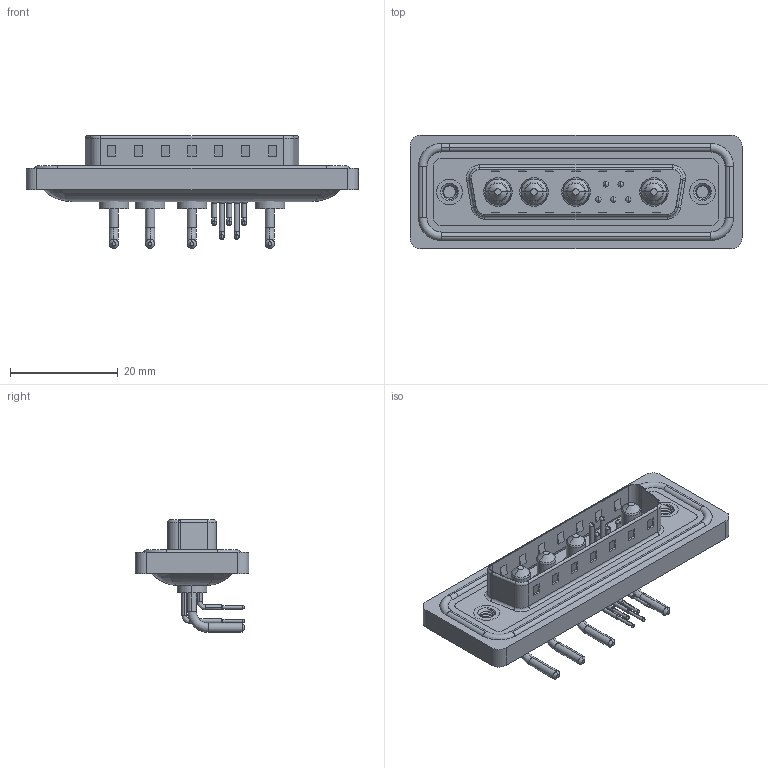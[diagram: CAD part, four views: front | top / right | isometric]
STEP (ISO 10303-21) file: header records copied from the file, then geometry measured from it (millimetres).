
FILE_DESCRIPTION (( 'STEP AP203' ), '1' );
FILE_NAME ('629W9W4-240-1N2.STEP', '2024-04-11T15:27:52', ( '' ), ( '' ), 'SwSTEP 2.0', 'SolidWorks 2023', '' );
FILE_SCHEMA (( 'CONFIG_CONTROL_DESIGN' ));
Length unit declared in the file: millimetre
Products named in the file (9): 629Combo Shell Front_25 Contacts; 629Combo Waterproof Housing_25 Contacts; 629Combo Threaded Rivet_2; 629Combo Shell Rear_25 Contacts; 629Combo Contact Row 1; 629Combo Housing_9W4; 629Combo Contact Row 2; Power Pin_10A RA; 629W9W4-240-1N2
Assembly tree (15 placements, depth 2):
  629W9W4-240-1N2
    629Combo Housing_9W4
    629Combo Shell Rear_25 Contacts
    629Combo Shell Front_25 Contacts
    629Combo Waterproof Housing_25 Contacts
    629Combo Threaded Rivet_2  x2
    Power Pin_10A RA  x4
    629Combo Contact Row 1  x2
    629Combo Contact Row 2  x3
Bounding box: 61.75 x 21.1 x 20.95 mm (x, y, z)
Volume: 7483.2 mm3; surface area: 12173.2 mm2
Topology: 20 solids, 20 shells, 1205 faces, 3159 edges, 2019 vertices
Faces by surface type: plane 569, cylinder 452, torus 80, cone 60, bspline 44
Entity records: 26116 total; most frequent: CARTESIAN_POINT 6065, DIRECTION 4074, ORIENTED_EDGE 3892, EDGE_CURVE 1946, AXIS2_PLACEMENT_3D 1449, VERTEX_POINT 1251, LINE 1176, VECTOR 1176
